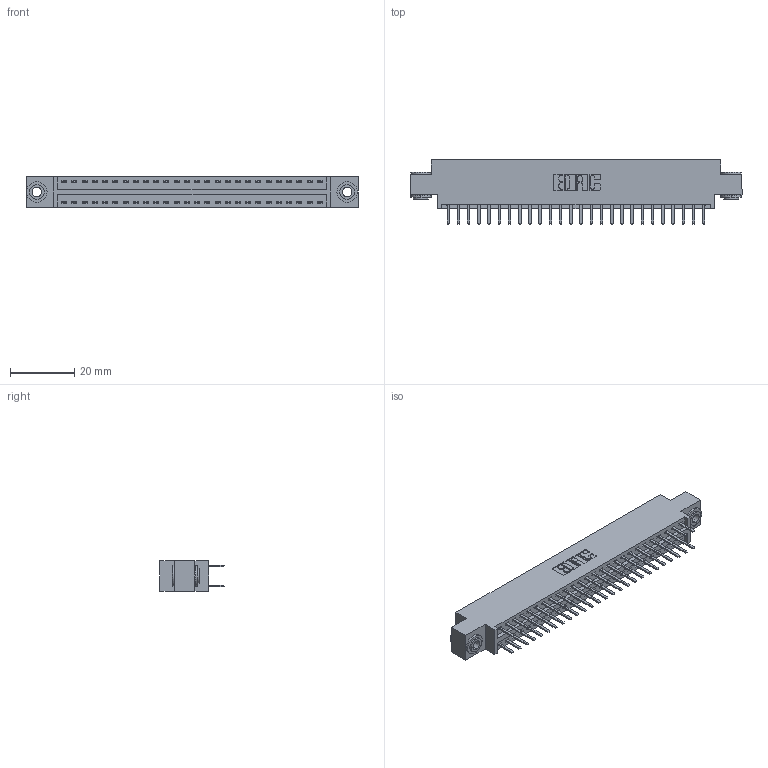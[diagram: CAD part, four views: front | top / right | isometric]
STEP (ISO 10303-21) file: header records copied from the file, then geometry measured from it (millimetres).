
FILE_DESCRIPTION (( 'STEP AP203' ), '1' );
FILE_NAME ('396-052-520-803.STEP', '2019-11-02T07:30:58', ( '' ), ( '' ), 'SwSTEP 2.0', 'SolidWorks 2016', '' );
FILE_SCHEMA (( 'CONFIG_CONTROL_DESIGN' ));
Length unit declared in the file: inch
Products named in the file (4): 346 Part_0.170 Offset - 0.156 Dia-TH; 345-292-001_345-293-120; 345-250-002_345-250-002-102; 396-052-520-803
Assembly tree (55 placements, depth 2):
  396-052-520-803
    346 Part_0.170 Offset - 0.156 Dia-TH
    345-292-001_345-293-120  x52
    345-250-002_345-250-002-102  x2
Bounding box: 103.12 x 20.02 x 9.4 mm (x, y, z)
Volume: 9773.5 mm3; surface area: 13523.1 mm2
Topology: 55 solids, 55 shells, 3076 faces, 8893 edges, 5786 vertices
Faces by surface type: plane 2014, cylinder 1054, cone 8
Entity records: 20018 total; most frequent: CARTESIAN_POINT 3311, ORIENTED_EDGE 3226, DIRECTION 2987, EDGE_CURVE 1613, LINE 1349, VECTOR 1349, VERTEX_POINT 1070, AXIS2_PLACEMENT_3D 819
